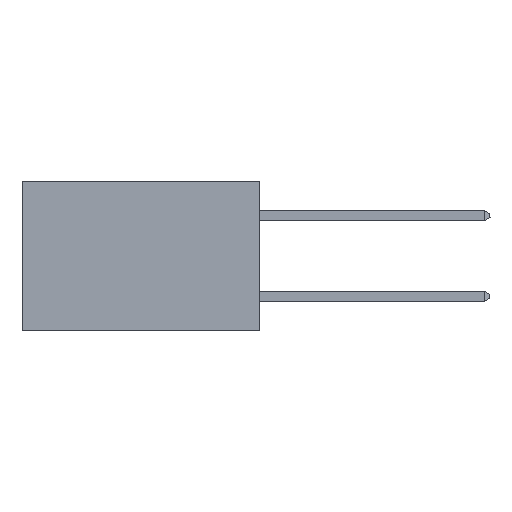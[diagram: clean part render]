
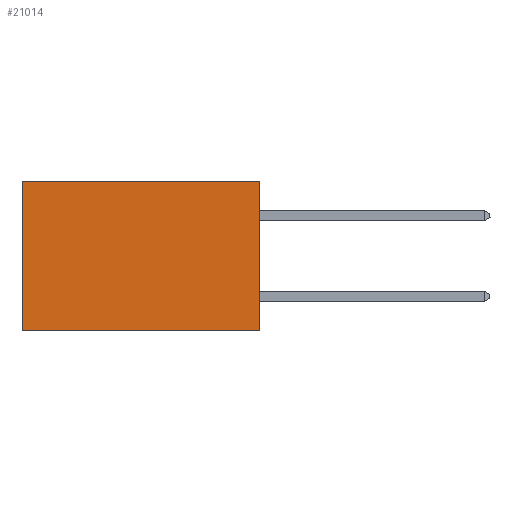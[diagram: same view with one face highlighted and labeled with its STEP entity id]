
A CAD part, left-side view. The second image highlights one B-rep face of the part: STEP entity #21014.
In plain terms, the highlighted planar face has unit normal (-1, 0, 0).
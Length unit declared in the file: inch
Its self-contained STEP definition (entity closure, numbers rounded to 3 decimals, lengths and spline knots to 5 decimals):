
#32 = EDGE_CURVE ( 'NONE', #25791, #6073, #17150, .T. ) ;
#1271 = CARTESIAN_POINT ( 'NONE',  ( 0.277, 0.59, -0.37 ) ) ;
#2678 = VECTOR ( 'NONE', #13505, 39.37008 ) ;
#3800 = DIRECTION ( 'NONE',  ( 0., 1., 0. ) ) ;
#5151 = CARTESIAN_POINT ( 'NONE',  ( 0.277, 0., -0.37 ) ) ;
#6073 = VERTEX_POINT ( 'NONE', #24347 ) ;
#6307 = VECTOR ( 'NONE', #3800, 39.37008 ) ;
#7199 = DIRECTION ( 'NONE',  ( 0., 0., -1. ) ) ;
#7478 = PLANE ( 'NONE',  #9656 ) ;
#7491 = CARTESIAN_POINT ( 'NONE',  ( 0.277, 0.59, -0.37 ) ) ;
#9526 = DIRECTION ( 'NONE',  ( 1., 0., 0. ) ) ;
#9656 = AXIS2_PLACEMENT_3D ( 'NONE', #19581, #9526, #23560 ) ;
#10255 = CARTESIAN_POINT ( 'NONE',  ( 0.277, 0., -0.37 ) ) ;
#10344 = VECTOR ( 'NONE', #22269, 39.37008 ) ;
#10916 = ORIENTED_EDGE ( 'NONE', *, *, #19199, .T. ) ;
#11065 = CARTESIAN_POINT ( 'NONE',  ( 0.277, 0., 0. ) ) ;
#11079 = ORIENTED_EDGE ( 'NONE', *, *, #32, .T. ) ;
#13505 = DIRECTION ( 'NONE',  ( 0., 0., -1. ) ) ;
#13562 = LINE ( 'NONE', #1271, #2678 ) ;
#13741 = CARTESIAN_POINT ( 'NONE',  ( 0.277, 0., -0.37 ) ) ;
#13918 = ORIENTED_EDGE ( 'NONE', *, *, #17551, .F. ) ;
#14108 = VECTOR ( 'NONE', #7199, 39.37008 ) ;
#14419 = CARTESIAN_POINT ( 'NONE',  ( 0.277, 0., 0. ) ) ;
#15776 = LINE ( 'NONE', #10255, #10344 ) ;
#17150 = LINE ( 'NONE', #14419, #6307 ) ;
#17332 = VERTEX_POINT ( 'NONE', #13741 ) ;
#17551 = EDGE_CURVE ( 'NONE', #17332, #18007, #15776, .T. ) ;
#18007 = VERTEX_POINT ( 'NONE', #7491 ) ;
#18180 = ORIENTED_EDGE ( 'NONE', *, *, #20940, .F. ) ;
#19199 = EDGE_CURVE ( 'NONE', #6073, #18007, #13562, .T. ) ;
#19581 = CARTESIAN_POINT ( 'NONE',  ( 0.277, 0., -0.37 ) ) ;
#20940 = EDGE_CURVE ( 'NONE', #25791, #17332, #24713, .T. ) ;
#21014 = ADVANCED_FACE ( 'NONE', ( #22178 ), #7478, .F. ) ;
#21979 = EDGE_LOOP ( 'NONE', ( #10916, #13918, #18180, #11079 ) ) ;
#22178 = FACE_OUTER_BOUND ( 'NONE', #21979, .T. ) ;
#22269 = DIRECTION ( 'NONE',  ( 0., 1., 0. ) ) ;
#23560 = DIRECTION ( 'NONE',  ( 0., 0., -1. ) ) ;
#24347 = CARTESIAN_POINT ( 'NONE',  ( 0.277, 0.59, 0. ) ) ;
#24713 = LINE ( 'NONE', #5151, #14108 ) ;
#25791 = VERTEX_POINT ( 'NONE', #11065 ) ;
